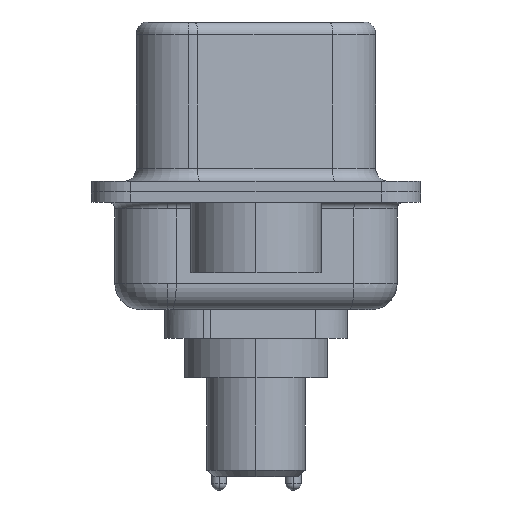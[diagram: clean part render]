
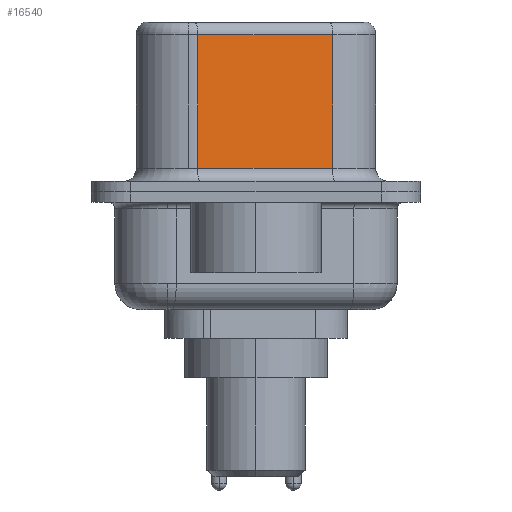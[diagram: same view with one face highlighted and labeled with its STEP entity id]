
A CAD part, left-side view. The second image highlights one B-rep face of the part: STEP entity #16540.
In plain terms, the highlighted planar face has unit normal (-0.985, -0.174, 0).
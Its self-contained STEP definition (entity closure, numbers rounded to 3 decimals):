
#191 = ORIENTED_EDGE ( 'NONE', *, *, #9408, .T. ) ;
#261 = CARTESIAN_POINT ( 'NONE',  ( 4.585, -2.927, 6.02 ) ) ;
#1215 = EDGE_CURVE ( 'NONE', #10539, #11317, #3714, .T. ) ;
#1799 = PLANE ( 'NONE',  #11972 ) ;
#1845 = CARTESIAN_POINT ( 'NONE',  ( 4.585, -2.927, 6.52 ) ) ;
#2006 = VECTOR ( 'NONE', #7553, 1000. ) ;
#2632 = DIRECTION ( 'NONE',  ( 0., 0., -1. ) ) ;
#3121 = EDGE_CURVE ( 'NONE', #8229, #11317, #9074, .T. ) ;
#3153 = DIRECTION ( 'NONE',  ( -0.174, 0.985, 0. ) ) ;
#3336 = CARTESIAN_POINT ( 'NONE',  ( 3.675, 2.233, 6.02 ) ) ;
#3448 = VECTOR ( 'NONE', #8292, 1000. ) ;
#3451 = CARTESIAN_POINT ( 'NONE',  ( 3.675, 2.233, 6.52 ) ) ;
#3714 = LINE ( 'NONE', #1845, #14277 ) ;
#5483 = CARTESIAN_POINT ( 'NONE',  ( 4.585, -2.927, 6.02 ) ) ;
#5851 = VECTOR ( 'NONE', #11385, 1000. ) ;
#7095 = CARTESIAN_POINT ( 'NONE',  ( 4.585, -2.927, 6.52 ) ) ;
#7553 = DIRECTION ( 'NONE',  ( 0.174, -0.985, 0. ) ) ;
#8051 = ORIENTED_EDGE ( 'NONE', *, *, #3121, .T. ) ;
#8229 = VERTEX_POINT ( 'NONE', #11964 ) ;
#8292 = DIRECTION ( 'NONE',  ( -0.174, 0.985, 0. ) ) ;
#8689 = CARTESIAN_POINT ( 'NONE',  ( 4.585, -2.927, 0.9 ) ) ;
#9074 = LINE ( 'NONE', #14213, #2006 ) ;
#9408 = EDGE_CURVE ( 'NONE', #10539, #12780, #14825, .T. ) ;
#9798 = EDGE_LOOP ( 'NONE', ( #9872, #191, #16360, #8051 ) ) ;
#9872 = ORIENTED_EDGE ( 'NONE', *, *, #1215, .F. ) ;
#10539 = VERTEX_POINT ( 'NONE', #5483 ) ;
#11085 = DIRECTION ( 'NONE',  ( 0.985, 0.174, 0. ) ) ;
#11317 = VERTEX_POINT ( 'NONE', #8689 ) ;
#11385 = DIRECTION ( 'NONE',  ( 0., 0., -1. ) ) ;
#11964 = CARTESIAN_POINT ( 'NONE',  ( 3.675, 2.233, 0.9 ) ) ;
#11972 = AXIS2_PLACEMENT_3D ( 'NONE', #7095, #11085, #3153 ) ;
#12483 = LINE ( 'NONE', #3451, #5851 ) ;
#12780 = VERTEX_POINT ( 'NONE', #3336 ) ;
#12838 = EDGE_CURVE ( 'NONE', #12780, #8229, #12483, .T. ) ;
#13205 = FACE_OUTER_BOUND ( 'NONE', #9798, .T. ) ;
#14213 = CARTESIAN_POINT ( 'NONE',  ( 4.585, -2.927, 0.9 ) ) ;
#14277 = VECTOR ( 'NONE', #2632, 1000. ) ;
#14825 = LINE ( 'NONE', #261, #3448 ) ;
#16360 = ORIENTED_EDGE ( 'NONE', *, *, #12838, .T. ) ;
#16540 = ADVANCED_FACE ( 'NONE', ( #13205 ), #1799, .F. ) ;
